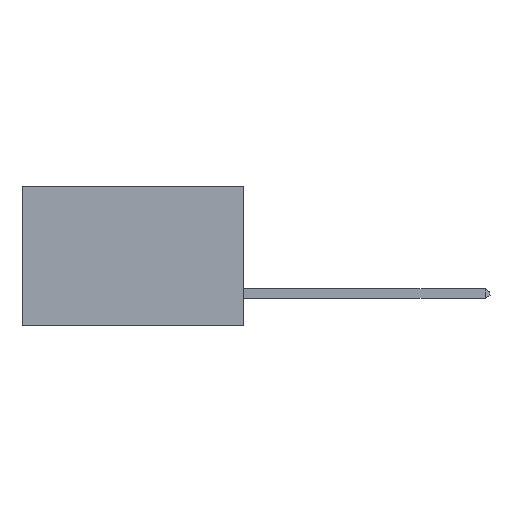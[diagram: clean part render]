
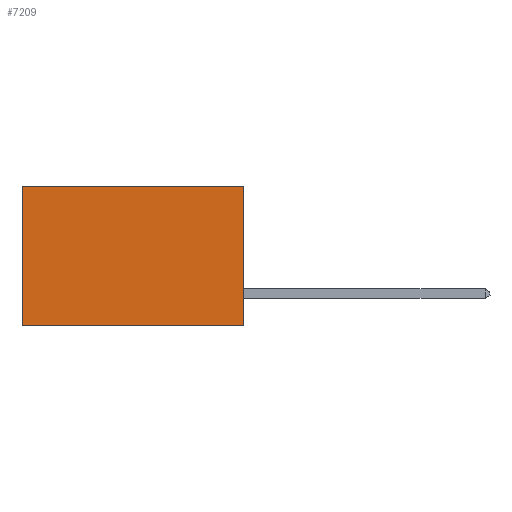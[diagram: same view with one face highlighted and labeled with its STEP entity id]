
A CAD part, left-side view. The second image highlights one B-rep face of the part: STEP entity #7209.
In plain terms, the highlighted planar face has unit normal (-1, 0, 0).
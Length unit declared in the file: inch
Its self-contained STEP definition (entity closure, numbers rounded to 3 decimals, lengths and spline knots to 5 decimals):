
#579 = CARTESIAN_POINT ( 'NONE',  ( 0.277, 0., -0.37 ) ) ;
#786 = EDGE_CURVE ( 'NONE', #9618, #9333, #1978, .T. ) ;
#849 = DIRECTION ( 'NONE',  ( 0., 1., 0. ) ) ;
#1570 = DIRECTION ( 'NONE',  ( 0., 0., -1. ) ) ;
#1571 = ORIENTED_EDGE ( 'NONE', *, *, #786, .F. ) ;
#1855 = CARTESIAN_POINT ( 'NONE',  ( 0.277, 0.59, -0.37 ) ) ;
#1895 = DIRECTION ( 'NONE',  ( 0., 0., -1. ) ) ;
#1978 = LINE ( 'NONE', #4575, #10494 ) ;
#2331 = VERTEX_POINT ( 'NONE', #4135 ) ;
#2413 = FACE_OUTER_BOUND ( 'NONE', #7212, .T. ) ;
#2507 = EDGE_CURVE ( 'NONE', #9333, #2331, #9746, .T. ) ;
#2667 = VERTEX_POINT ( 'NONE', #7074 ) ;
#2716 = CARTESIAN_POINT ( 'NONE',  ( 0.277, 0., -0.37 ) ) ;
#2881 = LINE ( 'NONE', #1855, #7127 ) ;
#3847 = CARTESIAN_POINT ( 'NONE',  ( 0.277, 0., 0. ) ) ;
#4135 = CARTESIAN_POINT ( 'NONE',  ( 0.277, 0.59, -0.37 ) ) ;
#4575 = CARTESIAN_POINT ( 'NONE',  ( 0.277, 0., -0.37 ) ) ;
#5065 = ORIENTED_EDGE ( 'NONE', *, *, #6882, .T. ) ;
#5316 = VECTOR ( 'NONE', #849, 39.37008 ) ;
#5544 = VECTOR ( 'NONE', #9744, 39.37008 ) ;
#6403 = DIRECTION ( 'NONE',  ( 0., 0., -1. ) ) ;
#6430 = DIRECTION ( 'NONE',  ( 1., 0., 0. ) ) ;
#6448 = PLANE ( 'NONE',  #10667 ) ;
#6708 = CARTESIAN_POINT ( 'NONE',  ( 0.277, 0., -0.37 ) ) ;
#6882 = EDGE_CURVE ( 'NONE', #9618, #2667, #10200, .T. ) ;
#7074 = CARTESIAN_POINT ( 'NONE',  ( 0.277, 0.59, 0. ) ) ;
#7127 = VECTOR ( 'NONE', #1895, 39.37008 ) ;
#7209 = ADVANCED_FACE ( 'NONE', ( #2413 ), #6448, .F. ) ;
#7212 = EDGE_LOOP ( 'NONE', ( #10072, #10100, #1571, #5065 ) ) ;
#8817 = EDGE_CURVE ( 'NONE', #2667, #2331, #2881, .T. ) ;
#9333 = VERTEX_POINT ( 'NONE', #2716 ) ;
#9618 = VERTEX_POINT ( 'NONE', #3847 ) ;
#9744 = DIRECTION ( 'NONE',  ( 0., 1., 0. ) ) ;
#9746 = LINE ( 'NONE', #579, #5316 ) ;
#9768 = CARTESIAN_POINT ( 'NONE',  ( 0.277, 0., 0. ) ) ;
#10072 = ORIENTED_EDGE ( 'NONE', *, *, #8817, .T. ) ;
#10100 = ORIENTED_EDGE ( 'NONE', *, *, #2507, .F. ) ;
#10200 = LINE ( 'NONE', #9768, #5544 ) ;
#10494 = VECTOR ( 'NONE', #1570, 39.37008 ) ;
#10667 = AXIS2_PLACEMENT_3D ( 'NONE', #6708, #6430, #6403 ) ;
